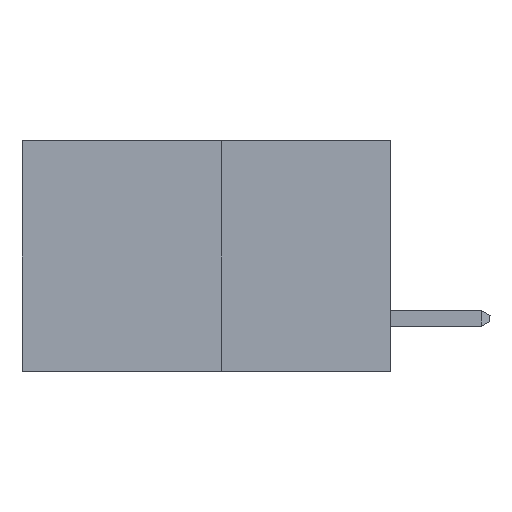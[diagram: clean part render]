
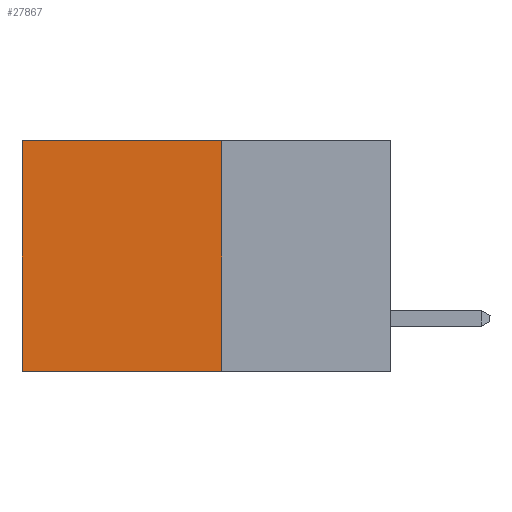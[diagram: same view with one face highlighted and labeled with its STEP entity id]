
A CAD part, left-side view. The second image highlights one B-rep face of the part: STEP entity #27867.
In plain terms, the highlighted planar face has unit normal (-1, 0, 0).
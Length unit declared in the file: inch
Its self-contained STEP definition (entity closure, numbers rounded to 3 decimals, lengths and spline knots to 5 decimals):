
#472 = VECTOR ( 'NONE', #5007, 39.37008 ) ;
#1179 = EDGE_CURVE ( 'NONE', #30272, #29847, #20723, .T. ) ;
#1251 = LINE ( 'NONE', #24875, #472 ) ;
#2739 = DIRECTION ( 'NONE',  ( 1., 0., 0. ) ) ;
#3396 = VECTOR ( 'NONE', #14895, 39.37008 ) ;
#3968 = CARTESIAN_POINT ( 'NONE',  ( 0.277, 0.27, 0. ) ) ;
#4290 = ORIENTED_EDGE ( 'NONE', *, *, #1179, .F. ) ;
#4873 = CARTESIAN_POINT ( 'NONE',  ( 0.277, 0.59, -0.37 ) ) ;
#5007 = DIRECTION ( 'NONE',  ( 0., 0., -1. ) ) ;
#6653 = LINE ( 'NONE', #22447, #13305 ) ;
#6830 = ORIENTED_EDGE ( 'NONE', *, *, #18846, .F. ) ;
#9419 = VERTEX_POINT ( 'NONE', #12499 ) ;
#11500 = ORIENTED_EDGE ( 'NONE', *, *, #23284, .T. ) ;
#11805 = ORIENTED_EDGE ( 'NONE', *, *, #21942, .T. ) ;
#12427 = CARTESIAN_POINT ( 'NONE',  ( 0.277, 0.27, 0. ) ) ;
#12499 = CARTESIAN_POINT ( 'NONE',  ( 0.277, 0.59, 0. ) ) ;
#12693 = PLANE ( 'NONE',  #28470 ) ;
#13305 = VECTOR ( 'NONE', #24825, 39.37008 ) ;
#14123 = VECTOR ( 'NONE', #16266, 39.37008 ) ;
#14895 = DIRECTION ( 'NONE',  ( 0., 1., 0. ) ) ;
#15852 = LINE ( 'NONE', #12427, #3396 ) ;
#16266 = DIRECTION ( 'NONE',  ( 0., 1., 0. ) ) ;
#17670 = CARTESIAN_POINT ( 'NONE',  ( 0.277, 0.27, -0.37 ) ) ;
#18846 = EDGE_CURVE ( 'NONE', #21003, #30272, #1251, .T. ) ;
#19163 = CARTESIAN_POINT ( 'NONE',  ( 0.277, 0.27, -0.37 ) ) ;
#20185 = DIRECTION ( 'NONE',  ( 0., 0., -1. ) ) ;
#20723 = LINE ( 'NONE', #19163, #14123 ) ;
#21003 = VERTEX_POINT ( 'NONE', #3968 ) ;
#21942 = EDGE_CURVE ( 'NONE', #21003, #9419, #15852, .T. ) ;
#22447 = CARTESIAN_POINT ( 'NONE',  ( 0.277, 0.59, -0.37 ) ) ;
#23161 = EDGE_LOOP ( 'NONE', ( #11500, #4290, #6830, #11805 ) ) ;
#23284 = EDGE_CURVE ( 'NONE', #9419, #29847, #6653, .T. ) ;
#23874 = FACE_OUTER_BOUND ( 'NONE', #23161, .T. ) ;
#24825 = DIRECTION ( 'NONE',  ( 0., 0., -1. ) ) ;
#24875 = CARTESIAN_POINT ( 'NONE',  ( 0.277, 0.27, -0.37 ) ) ;
#27867 = ADVANCED_FACE ( 'NONE', ( #23874 ), #12693, .F. ) ;
#28470 = AXIS2_PLACEMENT_3D ( 'NONE', #17670, #2739, #20185 ) ;
#28792 = CARTESIAN_POINT ( 'NONE',  ( 0.277, 0.27, -0.37 ) ) ;
#29847 = VERTEX_POINT ( 'NONE', #4873 ) ;
#30272 = VERTEX_POINT ( 'NONE', #28792 ) ;
